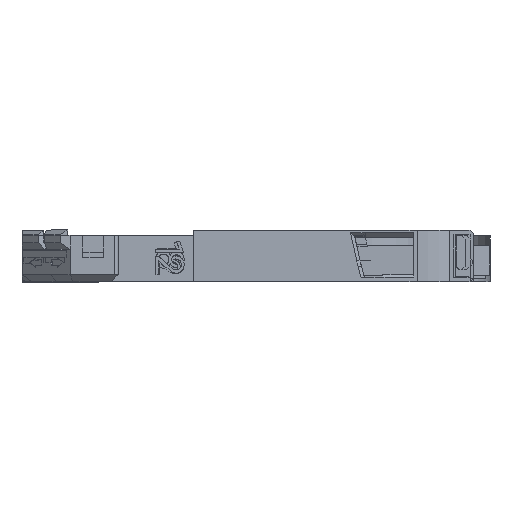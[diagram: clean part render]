
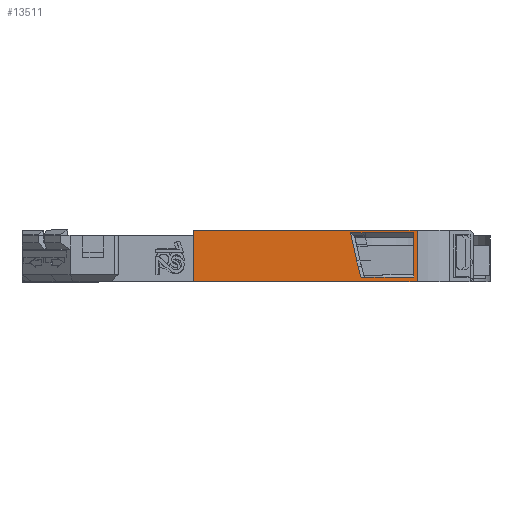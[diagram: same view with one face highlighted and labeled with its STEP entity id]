
A CAD part, top view. The second image highlights one B-rep face of the part: STEP entity #13511.
In plain terms, the highlighted planar face has unit normal (0, 0, 1).
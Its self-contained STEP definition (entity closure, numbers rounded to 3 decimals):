
#9211 = VERTEX_POINT('',#9212);
#9212 = CARTESIAN_POINT('',(0.,-15.,34.99));
#9218 = EDGE_CURVE('',#9211,#9219,#9221,.T.);
#9219 = VERTEX_POINT('',#9220);
#9220 = CARTESIAN_POINT('',(65.,-15.,34.99));
#9221 = LINE('',#9222,#9223);
#9222 = CARTESIAN_POINT('',(0.,-15.,34.99));
#9223 = VECTOR('',#9224,1.);
#9224 = DIRECTION('',(1.,0.,0.));
#12483 = VERTEX_POINT('',#12484);
#12484 = CARTESIAN_POINT('',(0.,0.,34.99));
#12490 = EDGE_CURVE('',#12483,#12491,#12493,.T.);
#12491 = VERTEX_POINT('',#12492);
#12492 = CARTESIAN_POINT('',(65.,0.,34.99));
#12493 = LINE('',#12494,#12495);
#12494 = CARTESIAN_POINT('',(0.,0.,34.99));
#12495 = VECTOR('',#12496,1.);
#12496 = DIRECTION('',(1.,0.,0.));
#13124 = VERTEX_POINT('',#13125);
#13125 = CARTESIAN_POINT('',(0.,-1.6,34.99));
#13131 = EDGE_CURVE('',#9211,#13124,#13132,.T.);
#13132 = LINE('',#13133,#13134);
#13133 = CARTESIAN_POINT('',(0.,-15.,34.99));
#13134 = VECTOR('',#13135,1.);
#13135 = DIRECTION('',(0.,1.,0.));
#13511 = ADVANCED_FACE('',(#13512,#13529),#13675,.F.);
#13512 = FACE_BOUND('',#13513,.F.);
#13513 = EDGE_LOOP('',(#13514,#13515,#13521,#13522,#13528));
#13514 = ORIENTED_EDGE('',*,*,#13131,.T.);
#13515 = ORIENTED_EDGE('',*,*,#13516,.T.);
#13516 = EDGE_CURVE('',#13124,#12483,#13517,.T.);
#13517 = LINE('',#13518,#13519);
#13518 = CARTESIAN_POINT('',(0.,-15.,34.99));
#13519 = VECTOR('',#13520,1.);
#13520 = DIRECTION('',(0.,1.,0.));
#13521 = ORIENTED_EDGE('',*,*,#12490,.T.);
#13522 = ORIENTED_EDGE('',*,*,#13523,.F.);
#13523 = EDGE_CURVE('',#9219,#12491,#13524,.T.);
#13524 = LINE('',#13525,#13526);
#13525 = CARTESIAN_POINT('',(65.,-15.,34.99));
#13526 = VECTOR('',#13527,1.);
#13527 = DIRECTION('',(0.,1.,0.));
#13528 = ORIENTED_EDGE('',*,*,#9218,.F.);
#13529 = FACE_BOUND('',#13530,.F.);
#13530 = EDGE_LOOP('',(#13531,#13541,#13549,#13557,#13565,#13573,#13581,
    #13589,#13597,#13605,#13613,#13621,#13629,#13637,#13645,#13653,
    #13661,#13669));
#13531 = ORIENTED_EDGE('',*,*,#13532,.F.);
#13532 = EDGE_CURVE('',#13533,#13535,#13537,.T.);
#13533 = VERTEX_POINT('',#13534);
#13534 = CARTESIAN_POINT('',(51.789,-13.75,34.99));
#13535 = VERTEX_POINT('',#13536);
#13536 = CARTESIAN_POINT('',(48.716,-13.75,34.99));
#13537 = LINE('',#13538,#13539);
#13538 = CARTESIAN_POINT('',(51.789,-13.75,34.99));
#13539 = VECTOR('',#13540,1.);
#13540 = DIRECTION('',(-1.,0.,-0.));
#13541 = ORIENTED_EDGE('',*,*,#13542,.T.);
#13542 = EDGE_CURVE('',#13533,#13543,#13545,.T.);
#13543 = VERTEX_POINT('',#13544);
#13544 = CARTESIAN_POINT('',(51.841,-13.75,34.99));
#13545 = LINE('',#13546,#13547);
#13546 = CARTESIAN_POINT('',(52.871,-13.75,34.99));
#13547 = VECTOR('',#13548,1.);
#13548 = DIRECTION('',(1.,0.,0.));
#13549 = ORIENTED_EDGE('',*,*,#13550,.F.);
#13550 = EDGE_CURVE('',#13551,#13543,#13553,.T.);
#13551 = VERTEX_POINT('',#13552);
#13552 = CARTESIAN_POINT('',(52.773,-13.75,34.99));
#13553 = LINE('',#13554,#13555);
#13554 = CARTESIAN_POINT('',(27.386,-13.75,34.99));
#13555 = VECTOR('',#13556,1.);
#13556 = DIRECTION('',(-1.,0.,-0.));
#13557 = ORIENTED_EDGE('',*,*,#13558,.F.);
#13558 = EDGE_CURVE('',#13559,#13551,#13561,.T.);
#13559 = VERTEX_POINT('',#13560);
#13560 = CARTESIAN_POINT('',(54.773,-13.75,34.99));
#13561 = LINE('',#13562,#13563);
#13562 = CARTESIAN_POINT('',(54.773,-13.75,34.99));
#13563 = VECTOR('',#13564,1.);
#13564 = DIRECTION('',(-1.,0.,0.));
#13565 = ORIENTED_EDGE('',*,*,#13566,.F.);
#13566 = EDGE_CURVE('',#13567,#13559,#13569,.T.);
#13567 = VERTEX_POINT('',#13568);
#13568 = CARTESIAN_POINT('',(54.791,-13.7,34.99));
#13569 = LINE('',#13570,#13571);
#13570 = CARTESIAN_POINT('',(55.046,-13.,34.99));
#13571 = VECTOR('',#13572,1.);
#13572 = DIRECTION('',(-0.342,-0.94,
    0.));
#13573 = ORIENTED_EDGE('',*,*,#13574,.F.);
#13574 = EDGE_CURVE('',#13575,#13567,#13577,.T.);
#13575 = VERTEX_POINT('',#13576);
#13576 = CARTESIAN_POINT('',(64.,-13.7,34.99));
#13577 = LINE('',#13578,#13579);
#13578 = CARTESIAN_POINT('',(64.,-13.7,34.99));
#13579 = VECTOR('',#13580,1.);
#13580 = DIRECTION('',(-1.,0.,0.));
#13581 = ORIENTED_EDGE('',*,*,#13582,.F.);
#13582 = EDGE_CURVE('',#13583,#13575,#13585,.T.);
#13583 = VERTEX_POINT('',#13584);
#13584 = CARTESIAN_POINT('',(64.,-13.,34.99));
#13585 = LINE('',#13586,#13587);
#13586 = CARTESIAN_POINT('',(64.,-12.,34.99));
#13587 = VECTOR('',#13588,1.);
#13588 = DIRECTION('',(0.,-1.,0.));
#13589 = ORIENTED_EDGE('',*,*,#13590,.F.);
#13590 = EDGE_CURVE('',#13591,#13583,#13593,.T.);
#13591 = VERTEX_POINT('',#13592);
#13592 = CARTESIAN_POINT('',(64.,-10.5,34.99));
#13593 = LINE('',#13594,#13595);
#13594 = CARTESIAN_POINT('',(64.,-9.,34.99));
#13595 = VECTOR('',#13596,1.);
#13596 = DIRECTION('',(0.,-1.,0.));
#13597 = ORIENTED_EDGE('',*,*,#13598,.F.);
#13598 = EDGE_CURVE('',#13599,#13591,#13601,.T.);
#13599 = VERTEX_POINT('',#13600);
#13600 = CARTESIAN_POINT('',(64.,-9.,34.99));
#13601 = LINE('',#13602,#13603);
#13602 = CARTESIAN_POINT('',(64.,-12.,34.99));
#13603 = VECTOR('',#13604,1.);
#13604 = DIRECTION('',(0.,-1.,0.));
#13605 = ORIENTED_EDGE('',*,*,#13606,.T.);
#13606 = EDGE_CURVE('',#13599,#13607,#13609,.T.);
#13607 = VERTEX_POINT('',#13608);
#13608 = CARTESIAN_POINT('',(64.,-2.25,34.99));
#13609 = LINE('',#13610,#13611);
#13610 = CARTESIAN_POINT('',(64.,-9.,34.99));
#13611 = VECTOR('',#13612,1.);
#13612 = DIRECTION('',(0.,1.,0.));
#13613 = ORIENTED_EDGE('',*,*,#13614,.T.);
#13614 = EDGE_CURVE('',#13607,#13615,#13617,.T.);
#13615 = VERTEX_POINT('',#13616);
#13616 = CARTESIAN_POINT('',(64.,-0.75,34.99));
#13617 = LINE('',#13618,#13619);
#13618 = CARTESIAN_POINT('',(64.,-12.,34.99));
#13619 = VECTOR('',#13620,1.);
#13620 = DIRECTION('',(0.,1.,0.));
#13621 = ORIENTED_EDGE('',*,*,#13622,.T.);
#13622 = EDGE_CURVE('',#13615,#13623,#13625,.T.);
#13623 = VERTEX_POINT('',#13624);
#13624 = CARTESIAN_POINT('',(50.,-0.75,34.99));
#13625 = LINE('',#13626,#13627);
#13626 = CARTESIAN_POINT('',(64.,-0.75,34.99));
#13627 = VECTOR('',#13628,1.);
#13628 = DIRECTION('',(-1.,0.,0.));
#13629 = ORIENTED_EDGE('',*,*,#13630,.T.);
#13630 = EDGE_CURVE('',#13623,#13631,#13633,.T.);
#13631 = VERTEX_POINT('',#13632);
#13632 = CARTESIAN_POINT('',(48.683,-0.75,34.99));
#13633 = LINE('',#13634,#13635);
#13634 = CARTESIAN_POINT('',(50.,-0.75,34.99));
#13635 = VECTOR('',#13636,1.);
#13636 = DIRECTION('',(-1.,0.,0.));
#13637 = ORIENTED_EDGE('',*,*,#13638,.T.);
#13638 = EDGE_CURVE('',#13631,#13639,#13641,.T.);
#13639 = VERTEX_POINT('',#13640);
#13640 = CARTESIAN_POINT('',(48.642,-0.75,34.99));
#13641 = LINE('',#13642,#13643);
#13642 = CARTESIAN_POINT('',(50.,-0.75,34.99));
#13643 = VECTOR('',#13644,1.);
#13644 = DIRECTION('',(-1.,0.,0.));
#13645 = ORIENTED_EDGE('',*,*,#13646,.T.);
#13646 = EDGE_CURVE('',#13639,#13647,#13649,.T.);
#13647 = VERTEX_POINT('',#13648);
#13648 = CARTESIAN_POINT('',(45.61,-0.75,34.99));
#13649 = LINE('',#13650,#13651);
#13650 = CARTESIAN_POINT('',(48.683,-0.75,34.99));
#13651 = VECTOR('',#13652,1.);
#13652 = DIRECTION('',(-1.,0.,-0.));
#13653 = ORIENTED_EDGE('',*,*,#13654,.F.);
#13654 = EDGE_CURVE('',#13655,#13647,#13657,.T.);
#13655 = VERTEX_POINT('',#13656);
#13656 = CARTESIAN_POINT('',(47.443,-9.,34.99));
#13657 = LINE('',#13658,#13659);
#13658 = CARTESIAN_POINT('',(47.443,-9.,34.99));
#13659 = VECTOR('',#13660,1.);
#13660 = DIRECTION('',(-0.217,0.976,
    0.));
#13661 = ORIENTED_EDGE('',*,*,#13662,.T.);
#13662 = EDGE_CURVE('',#13655,#13663,#13665,.T.);
#13663 = VERTEX_POINT('',#13664);
#13664 = CARTESIAN_POINT('',(47.845,-10.5,34.99));
#13665 = LINE('',#13666,#13667);
#13666 = CARTESIAN_POINT('',(47.509,-9.246,34.99));
#13667 = VECTOR('',#13668,1.);
#13668 = DIRECTION('',(0.259,-0.966,0.
    ));
#13669 = ORIENTED_EDGE('',*,*,#13670,.T.);
#13670 = EDGE_CURVE('',#13663,#13535,#13671,.T.);
#13671 = LINE('',#13672,#13673);
#13672 = CARTESIAN_POINT('',(47.845,-10.5,34.99));
#13673 = VECTOR('',#13674,1.);
#13674 = DIRECTION('',(0.259,-0.966,0.
    ));
#13675 = PLANE('',#13676);
#13676 = AXIS2_PLACEMENT_3D('',#13677,#13678,#13679);
#13677 = CARTESIAN_POINT('',(0.,-15.,34.99));
#13678 = DIRECTION('',(0.,0.,-1.));
#13679 = DIRECTION('',(1.,0.,0.));
